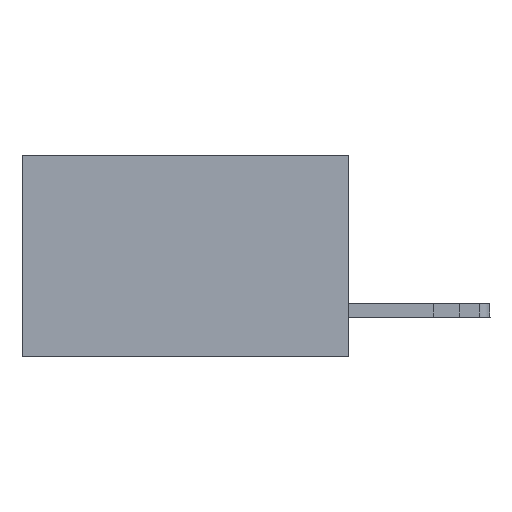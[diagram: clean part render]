
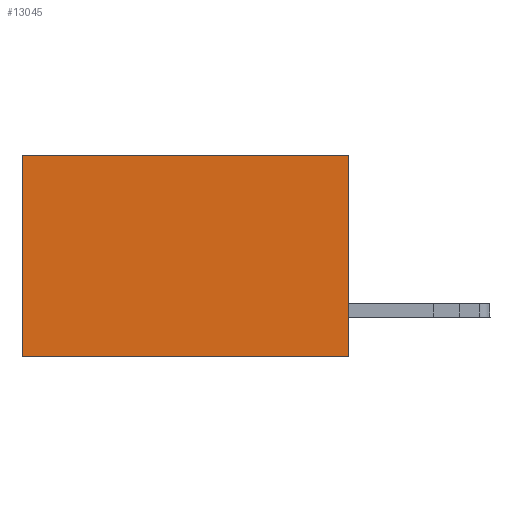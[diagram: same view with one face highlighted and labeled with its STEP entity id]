
A CAD part, left-side view. The second image highlights one B-rep face of the part: STEP entity #13045.
In plain terms, the highlighted planar face has unit normal (-1, 0, 0).
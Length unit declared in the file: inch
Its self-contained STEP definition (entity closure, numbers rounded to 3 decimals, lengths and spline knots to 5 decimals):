
#286 = DIRECTION ( 'NONE',  ( 0., 0., -1. ) ) ;
#889 = CARTESIAN_POINT ( 'NONE',  ( 0.298, 0., 0. ) ) ;
#1400 = DIRECTION ( 'NONE',  ( 0., 1., 0. ) ) ;
#1475 = DIRECTION ( 'NONE',  ( 0., 0., -1. ) ) ;
#2941 = CARTESIAN_POINT ( 'NONE',  ( 0.298, 0., -0.37 ) ) ;
#3350 = LINE ( 'NONE', #11176, #5963 ) ;
#3512 = VERTEX_POINT ( 'NONE', #22875 ) ;
#3816 = ORIENTED_EDGE ( 'NONE', *, *, #6354, .F. ) ;
#4816 = PLANE ( 'NONE',  #16578 ) ;
#5159 = EDGE_CURVE ( 'NONE', #3512, #14166, #12920, .T. ) ;
#5300 = VECTOR ( 'NONE', #1475, 39.37008 ) ;
#5963 = VECTOR ( 'NONE', #1400, 39.37008 ) ;
#6354 = EDGE_CURVE ( 'NONE', #21522, #14166, #7410, .T. ) ;
#6919 = EDGE_CURVE ( 'NONE', #13514, #21522, #11856, .T. ) ;
#7282 = CARTESIAN_POINT ( 'NONE',  ( 0.298, 0., -0.37 ) ) ;
#7410 = LINE ( 'NONE', #7282, #22774 ) ;
#8470 = ORIENTED_EDGE ( 'NONE', *, *, #5159, .T. ) ;
#8795 = CARTESIAN_POINT ( 'NONE',  ( 0.298, 0., 0. ) ) ;
#9792 = CARTESIAN_POINT ( 'NONE',  ( 0.298, 0., 0. ) ) ;
#11176 = CARTESIAN_POINT ( 'NONE',  ( 0.298, 0., 0. ) ) ;
#11769 = CARTESIAN_POINT ( 'NONE',  ( 0.298, 0.6, -0.37 ) ) ;
#11856 = LINE ( 'NONE', #9792, #23079 ) ;
#12645 = DIRECTION ( 'NONE',  ( 1., 0., 0. ) ) ;
#12920 = LINE ( 'NONE', #17174, #5300 ) ;
#13045 = ADVANCED_FACE ( 'NONE', ( #22390 ), #4816, .F. ) ;
#13514 = VERTEX_POINT ( 'NONE', #889 ) ;
#14166 = VERTEX_POINT ( 'NONE', #11769 ) ;
#14794 = DIRECTION ( 'NONE',  ( 0., 0., -1. ) ) ;
#14956 = EDGE_CURVE ( 'NONE', #13514, #3512, #3350, .T. ) ;
#16578 = AXIS2_PLACEMENT_3D ( 'NONE', #8795, #12645, #14794 ) ;
#17174 = CARTESIAN_POINT ( 'NONE',  ( 0.298, 0.6, 0. ) ) ;
#17438 = DIRECTION ( 'NONE',  ( 0., 1., 0. ) ) ;
#21194 = ORIENTED_EDGE ( 'NONE', *, *, #6919, .F. ) ;
#21522 = VERTEX_POINT ( 'NONE', #2941 ) ;
#22224 = ORIENTED_EDGE ( 'NONE', *, *, #14956, .T. ) ;
#22390 = FACE_OUTER_BOUND ( 'NONE', #24130, .T. ) ;
#22774 = VECTOR ( 'NONE', #17438, 39.37008 ) ;
#22875 = CARTESIAN_POINT ( 'NONE',  ( 0.298, 0.6, 0. ) ) ;
#23079 = VECTOR ( 'NONE', #286, 39.37008 ) ;
#24130 = EDGE_LOOP ( 'NONE', ( #8470, #3816, #21194, #22224 ) ) ;
